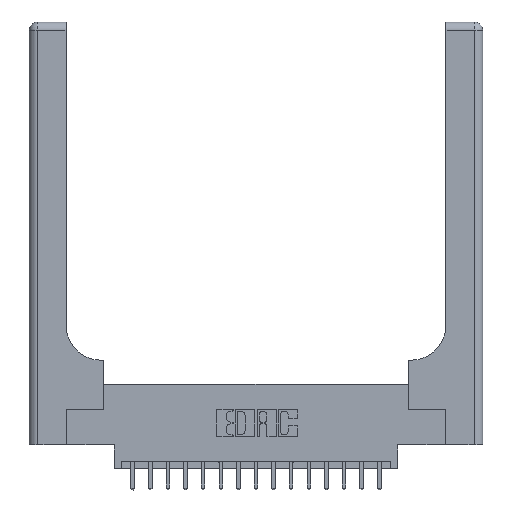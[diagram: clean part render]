
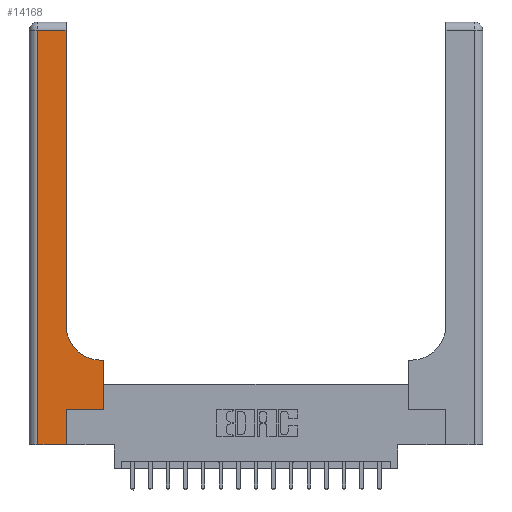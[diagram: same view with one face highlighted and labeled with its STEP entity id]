
A CAD part, top view. The second image highlights one B-rep face of the part: STEP entity #14168.
In plain terms, the highlighted planar face has unit normal (0, 0, 1).
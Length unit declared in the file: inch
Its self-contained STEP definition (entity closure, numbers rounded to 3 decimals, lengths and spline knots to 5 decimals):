
#791 = CARTESIAN_POINT ( 'NONE',  ( 0.528, 0.6, 0.37 ) ) ;
#793 = LINE ( 'NONE', #8318, #4207 ) ;
#806 = CARTESIAN_POINT ( 'NONE',  ( 0.265, 0.25, 0.37 ) ) ;
#1160 = PLANE ( 'NONE',  #6993 ) ;
#1169 = EDGE_LOOP ( 'NONE', ( #13877, #1656, #11679, #12582, #10741, #10780, #12188, #5287, #7565 ) ) ;
#1224 = DIRECTION ( 'NONE',  ( -1., 0., 0. ) ) ;
#1521 = VECTOR ( 'NONE', #3686, 39.37008 ) ;
#1593 = VERTEX_POINT ( 'NONE', #5206 ) ;
#1656 = ORIENTED_EDGE ( 'NONE', *, *, #4054, .T. ) ;
#1667 = VERTEX_POINT ( 'NONE', #16931 ) ;
#2249 = LINE ( 'NONE', #9327, #6614 ) ;
#2458 = DIRECTION ( 'NONE',  ( 0., -1., 0. ) ) ;
#2772 = DIRECTION ( 'NONE',  ( 1., 0., 0. ) ) ;
#3389 = VECTOR ( 'NONE', #13956, 39.37008 ) ;
#3593 = EDGE_CURVE ( 'NONE', #4627, #17797, #793, .T. ) ;
#3686 = DIRECTION ( 'NONE',  ( 0., 1., 0. ) ) ;
#3762 = CARTESIAN_POINT ( 'NONE',  ( 0.265, 0.25, 0.37 ) ) ;
#3839 = CARTESIAN_POINT ( 'NONE',  ( 0.26, 0.6, 0.37 ) ) ;
#4054 = EDGE_CURVE ( 'NONE', #14451, #4627, #5118, .T. ) ;
#4207 = VECTOR ( 'NONE', #2458, 39.37008 ) ;
#4627 = VERTEX_POINT ( 'NONE', #10693 ) ;
#5118 = LINE ( 'NONE', #15245, #12426 ) ;
#5206 = CARTESIAN_POINT ( 'NONE',  ( 0.51, 0.6, 0.37 ) ) ;
#5221 = LINE ( 'NONE', #8371, #16356 ) ;
#5257 = VECTOR ( 'NONE', #15488, 39.37008 ) ;
#5287 = ORIENTED_EDGE ( 'NONE', *, *, #6742, .T. ) ;
#5317 = VERTEX_POINT ( 'NONE', #3762 ) ;
#6614 = VECTOR ( 'NONE', #10744, 39.37008 ) ;
#6742 = EDGE_CURVE ( 'NONE', #13972, #1593, #16825, .T. ) ;
#6993 = AXIS2_PLACEMENT_3D ( 'NONE', #18585, #10013, #1224 ) ;
#7565 = ORIENTED_EDGE ( 'NONE', *, *, #15193, .T. ) ;
#7696 = EDGE_CURVE ( 'NONE', #10813, #5317, #2249, .T. ) ;
#7784 = CARTESIAN_POINT ( 'NONE',  ( 0.26, 2.94, 0.37 ) ) ;
#7846 = EDGE_CURVE ( 'NONE', #5317, #11787, #18759, .T. ) ;
#8273 = CARTESIAN_POINT ( 'NONE',  ( 0.51, 0.85, 0.37 ) ) ;
#8318 = CARTESIAN_POINT ( 'NONE',  ( 0.06, 3., 0.37 ) ) ;
#8371 = CARTESIAN_POINT ( 'NONE',  ( 0.26, 3., 0.37 ) ) ;
#9077 = VECTOR ( 'NONE', #2772, 39.37008 ) ;
#9327 = CARTESIAN_POINT ( 'NONE',  ( 0.265, 0., 0.37 ) ) ;
#9477 = FACE_OUTER_BOUND ( 'NONE', #1169, .T. ) ;
#9720 = DIRECTION ( 'NONE',  ( 1., 0., 0. ) ) ;
#10013 = DIRECTION ( 'NONE',  ( 0., 0., -1. ) ) ;
#10528 = EDGE_CURVE ( 'NONE', #1667, #14451, #5221, .T. ) ;
#10693 = CARTESIAN_POINT ( 'NONE',  ( 0.06, 2.94, 0.37 ) ) ;
#10741 = ORIENTED_EDGE ( 'NONE', *, *, #7696, .T. ) ;
#10744 = DIRECTION ( 'NONE',  ( 0., 1., 0. ) ) ;
#10780 = ORIENTED_EDGE ( 'NONE', *, *, #7846, .T. ) ;
#10813 = VERTEX_POINT ( 'NONE', #16508 ) ;
#10961 = DIRECTION ( 'NONE',  ( -1., 0., 0. ) ) ;
#11679 = ORIENTED_EDGE ( 'NONE', *, *, #3593, .T. ) ;
#11787 = VERTEX_POINT ( 'NONE', #12022 ) ;
#12022 = CARTESIAN_POINT ( 'NONE',  ( 0.528, 0.25, 0.37 ) ) ;
#12188 = ORIENTED_EDGE ( 'NONE', *, *, #12506, .T. ) ;
#12426 = VECTOR ( 'NONE', #10961, 39.37008 ) ;
#12506 = EDGE_CURVE ( 'NONE', #11787, #13972, #16540, .T. ) ;
#12582 = ORIENTED_EDGE ( 'NONE', *, *, #18283, .T. ) ;
#12702 = AXIS2_PLACEMENT_3D ( 'NONE', #8273, #18288, #9720 ) ;
#12939 = LINE ( 'NONE', #15752, #9077 ) ;
#13380 = CARTESIAN_POINT ( 'NONE',  ( 0.06, 0., 0.37 ) ) ;
#13877 = ORIENTED_EDGE ( 'NONE', *, *, #10528, .T. ) ;
#13956 = DIRECTION ( 'NONE',  ( 1., 0., 0. ) ) ;
#13972 = VERTEX_POINT ( 'NONE', #791 ) ;
#14168 = ADVANCED_FACE ( 'NONE', ( #9477 ), #1160, .F. ) ;
#14451 = VERTEX_POINT ( 'NONE', #7784 ) ;
#15193 = EDGE_CURVE ( 'NONE', #1593, #1667, #16224, .T. ) ;
#15245 = CARTESIAN_POINT ( 'NONE',  ( 0., 2.94, 0.37 ) ) ;
#15488 = DIRECTION ( 'NONE',  ( -1., 0., 0. ) ) ;
#15575 = DIRECTION ( 'NONE',  ( 0., 1., 0. ) ) ;
#15752 = CARTESIAN_POINT ( 'NONE',  ( 0., 0., 0.37 ) ) ;
#16224 = CIRCLE ( 'NONE', #12702, 0.25 ) ;
#16356 = VECTOR ( 'NONE', #15575, 39.37008 ) ;
#16508 = CARTESIAN_POINT ( 'NONE',  ( 0.265, 0., 0.37 ) ) ;
#16540 = LINE ( 'NONE', #18115, #1521 ) ;
#16825 = LINE ( 'NONE', #3839, #5257 ) ;
#16931 = CARTESIAN_POINT ( 'NONE',  ( 0.26, 0.85, 0.37 ) ) ;
#17797 = VERTEX_POINT ( 'NONE', #13380 ) ;
#18115 = CARTESIAN_POINT ( 'NONE',  ( 0.528, 0.25, 0.37 ) ) ;
#18283 = EDGE_CURVE ( 'NONE', #17797, #10813, #12939, .T. ) ;
#18288 = DIRECTION ( 'NONE',  ( 0., 0., -1. ) ) ;
#18585 = CARTESIAN_POINT ( 'NONE',  ( 0., 3., 0.37 ) ) ;
#18759 = LINE ( 'NONE', #806, #3389 ) ;
